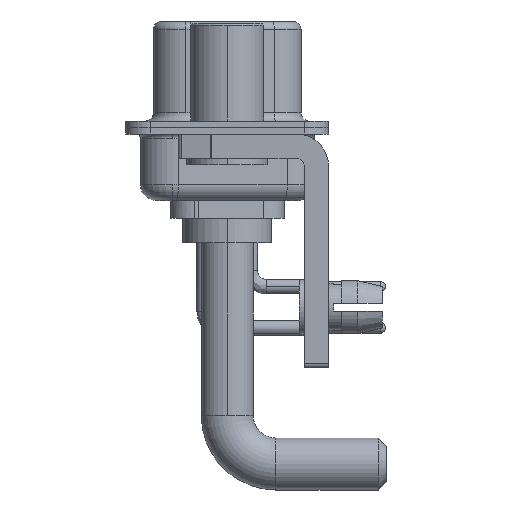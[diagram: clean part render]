
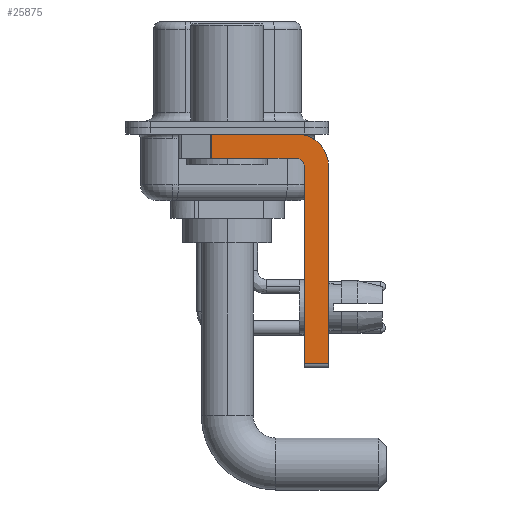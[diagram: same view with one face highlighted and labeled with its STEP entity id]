
A CAD part, left-side view. The second image highlights one B-rep face of the part: STEP entity #25875.
In plain terms, the highlighted planar face has unit normal (-1, 0, 0).
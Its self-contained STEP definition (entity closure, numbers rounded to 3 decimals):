
#106 = EDGE_CURVE ( 'NONE', #4652, #14262, #9776, .T. ) ;
#1149 = DIRECTION ( 'NONE',  ( 0., 0., -1. ) ) ;
#1378 = PLANE ( 'NONE',  #7501 ) ;
#1975 = VERTEX_POINT ( 'NONE', #4783 ) ;
#2190 = VERTEX_POINT ( 'NONE', #5362 ) ;
#2318 = EDGE_CURVE ( 'NONE', #2190, #7772, #12996, .T. ) ;
#3303 = LINE ( 'NONE', #21306, #14181 ) ;
#3320 = CARTESIAN_POINT ( 'NONE',  ( -2.9, -4.75, -2.4 ) ) ;
#4196 = FACE_OUTER_BOUND ( 'NONE', #27675, .T. ) ;
#4222 = ORIENTED_EDGE ( 'NONE', *, *, #2318, .T. ) ;
#4652 = VERTEX_POINT ( 'NONE', #10710 ) ;
#4783 = CARTESIAN_POINT ( 'NONE',  ( -2.9, -4.25, -0.4 ) ) ;
#4948 = EDGE_CURVE ( 'NONE', #22817, #4652, #24978, .T. ) ;
#5362 = CARTESIAN_POINT ( 'NONE',  ( -2.9, -4.75, -14.55 ) ) ;
#6076 = VECTOR ( 'NONE', #15511, 1000. ) ;
#6423 = CARTESIAN_POINT ( 'NONE',  ( -2.9, 0.978, -1.9 ) ) ;
#6457 = VECTOR ( 'NONE', #11067, 1000. ) ;
#7501 = AXIS2_PLACEMENT_3D ( 'NONE', #13023, #22173, #8170 ) ;
#7772 = VERTEX_POINT ( 'NONE', #16989 ) ;
#7947 = EDGE_CURVE ( 'NONE', #12345, #7772, #22165, .T. ) ;
#7957 = ORIENTED_EDGE ( 'NONE', *, *, #22543, .F. ) ;
#8170 = DIRECTION ( 'NONE',  ( 0., 0., -1. ) ) ;
#8357 = ORIENTED_EDGE ( 'NONE', *, *, #106, .F. ) ;
#9137 = CARTESIAN_POINT ( 'NONE',  ( -2.9, -6.25, -2.4 ) ) ;
#9776 = LINE ( 'NONE', #11863, #22244 ) ;
#10085 = DIRECTION ( 'NONE',  ( 0., 0., 1. ) ) ;
#10431 = CARTESIAN_POINT ( 'NONE',  ( -2.9, -4.25, -2.4 ) ) ;
#10710 = CARTESIAN_POINT ( 'NONE',  ( -2.9, -4.25, -1.9 ) ) ;
#11067 = DIRECTION ( 'NONE',  ( 0., -1., 0. ) ) ;
#11336 = EDGE_CURVE ( 'NONE', #2190, #22817, #27064, .T. ) ;
#11464 = EDGE_CURVE ( 'NONE', #19308, #1975, #3303, .T. ) ;
#11863 = CARTESIAN_POINT ( 'NONE',  ( -2.9, -4.25, -1.9 ) ) ;
#12310 = DIRECTION ( 'NONE',  ( -1., 0., 0. ) ) ;
#12345 = VERTEX_POINT ( 'NONE', #9137 ) ;
#12996 = LINE ( 'NONE', #26417, #6457 ) ;
#13023 = CARTESIAN_POINT ( 'NONE',  ( -2.9, -4.25, -2.4 ) ) ;
#13156 = DIRECTION ( 'NONE',  ( 0., 0., -1. ) ) ;
#14181 = VECTOR ( 'NONE', #20712, 1000. ) ;
#14262 = VERTEX_POINT ( 'NONE', #6423 ) ;
#15511 = DIRECTION ( 'NONE',  ( 0., 0., -1. ) ) ;
#15801 = LINE ( 'NONE', #24811, #6076 ) ;
#16132 = CARTESIAN_POINT ( 'NONE',  ( -2.9, -4.75, -14.8 ) ) ;
#16484 = AXIS2_PLACEMENT_3D ( 'NONE', #19232, #12310, #10085 ) ;
#16636 = DIRECTION ( 'NONE',  ( 1., 0., 0. ) ) ;
#16945 = VECTOR ( 'NONE', #13156, 1000. ) ;
#16989 = CARTESIAN_POINT ( 'NONE',  ( -2.9, -6.25, -14.55 ) ) ;
#17294 = CARTESIAN_POINT ( 'NONE',  ( -2.9, -6.25, -2.4 ) ) ;
#17374 = ORIENTED_EDGE ( 'NONE', *, *, #11336, .F. ) ;
#17948 = ORIENTED_EDGE ( 'NONE', *, *, #11464, .F. ) ;
#19232 = CARTESIAN_POINT ( 'NONE',  ( -2.9, -4.25, -2.4 ) ) ;
#19308 = VERTEX_POINT ( 'NONE', #20929 ) ;
#19430 = ORIENTED_EDGE ( 'NONE', *, *, #24184, .T. ) ;
#20712 = DIRECTION ( 'NONE',  ( 0., -1., 0. ) ) ;
#20929 = CARTESIAN_POINT ( 'NONE',  ( -2.9, 0.978, -0.4 ) ) ;
#21306 = CARTESIAN_POINT ( 'NONE',  ( -2.9, 3., -0.4 ) ) ;
#22165 = LINE ( 'NONE', #17294, #16945 ) ;
#22173 = DIRECTION ( 'NONE',  ( 1., 0., 0. ) ) ;
#22244 = VECTOR ( 'NONE', #22653, 1000. ) ;
#22466 = CIRCLE ( 'NONE', #24333, 2. ) ;
#22543 = EDGE_CURVE ( 'NONE', #1975, #12345, #22466, .T. ) ;
#22653 = DIRECTION ( 'NONE',  ( 0., 1., 0. ) ) ;
#22817 = VERTEX_POINT ( 'NONE', #3320 ) ;
#24069 = VECTOR ( 'NONE', #24855, 1000. ) ;
#24184 = EDGE_CURVE ( 'NONE', #19308, #14262, #15801, .T. ) ;
#24333 = AXIS2_PLACEMENT_3D ( 'NONE', #10431, #16636, #1149 ) ;
#24811 = CARTESIAN_POINT ( 'NONE',  ( -2.9, 0.978, -1.9 ) ) ;
#24855 = DIRECTION ( 'NONE',  ( 0., 0., 1. ) ) ;
#24978 = CIRCLE ( 'NONE', #16484, 0.5 ) ;
#25875 = ADVANCED_FACE ( 'NONE', ( #4196 ), #1378, .F. ) ;
#26417 = CARTESIAN_POINT ( 'NONE',  ( -2.9, -4.25, -14.55 ) ) ;
#27064 = LINE ( 'NONE', #16132, #24069 ) ;
#27675 = EDGE_LOOP ( 'NONE', ( #17948, #19430, #8357, #28228, #17374, #4222, #28380, #7957 ) ) ;
#28228 = ORIENTED_EDGE ( 'NONE', *, *, #4948, .F. ) ;
#28380 = ORIENTED_EDGE ( 'NONE', *, *, #7947, .F. ) ;
